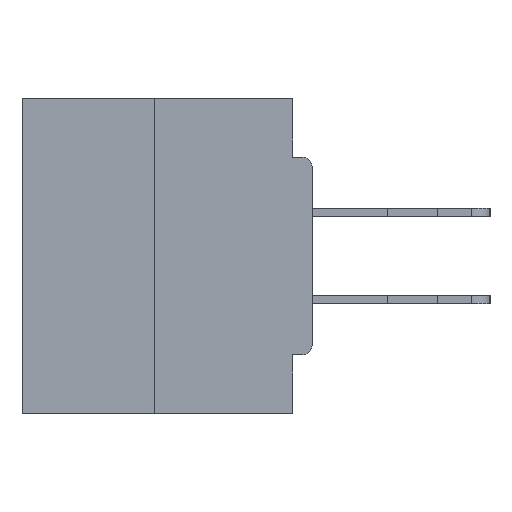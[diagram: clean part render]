
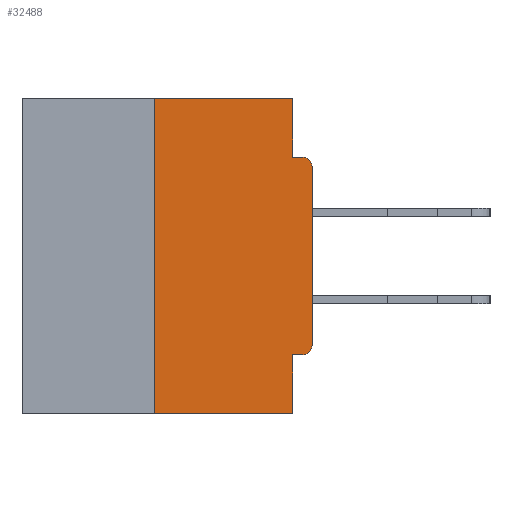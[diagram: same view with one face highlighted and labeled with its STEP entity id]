
A CAD part, left-side view. The second image highlights one B-rep face of the part: STEP entity #32488.
In plain terms, the highlighted planar face has unit normal (-1, 0, 0).
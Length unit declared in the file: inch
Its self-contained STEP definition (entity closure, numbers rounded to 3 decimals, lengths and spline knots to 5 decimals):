
#853 = FACE_OUTER_BOUND ( 'NONE', #29812, .T. ) ;
#1181 = VECTOR ( 'NONE', #7171, 39.37008 ) ;
#1456 = DIRECTION ( 'NONE',  ( 1., 0., 0. ) ) ;
#1654 = LINE ( 'NONE', #13604, #20247 ) ;
#1739 = CARTESIAN_POINT ( 'NONE',  ( 0., 0., 0. ) ) ;
#1899 = VECTOR ( 'NONE', #14951, 39.37008 ) ;
#1932 = VECTOR ( 'NONE', #18897, 39.37008 ) ;
#2019 = ORIENTED_EDGE ( 'NONE', *, *, #27860, .T. ) ;
#2384 = CARTESIAN_POINT ( 'NONE',  ( 0., 0.031, 0. ) ) ;
#3066 = CARTESIAN_POINT ( 'NONE',  ( 0., 0., -0.0935 ) ) ;
#3113 = CARTESIAN_POINT ( 'NONE',  ( 0., 0.015, -0.0935 ) ) ;
#3403 = ORIENTED_EDGE ( 'NONE', *, *, #8009, .T. ) ;
#4052 = ORIENTED_EDGE ( 'NONE', *, *, #5361, .F. ) ;
#4895 = VERTEX_POINT ( 'NONE', #2384 ) ;
#4952 = VECTOR ( 'NONE', #25074, 39.37008 ) ;
#5238 = VECTOR ( 'NONE', #13151, 39.37008 ) ;
#5361 = EDGE_CURVE ( 'NONE', #12038, #23537, #13809, .T. ) ;
#5390 = ORIENTED_EDGE ( 'NONE', *, *, #16022, .T. ) ;
#5860 = AXIS2_PLACEMENT_3D ( 'NONE', #29175, #13803, #16072 ) ;
#5918 = CARTESIAN_POINT ( 'NONE',  ( 0., 0.031, -0.4065 ) ) ;
#7171 = DIRECTION ( 'NONE',  ( 0., 1., 0. ) ) ;
#7186 = VERTEX_POINT ( 'NONE', #13687 ) ;
#7511 = ORIENTED_EDGE ( 'NONE', *, *, #31062, .F. ) ;
#7929 = CIRCLE ( 'NONE', #12005, 0.015 ) ;
#8009 = EDGE_CURVE ( 'NONE', #15146, #13964, #25191, .T. ) ;
#8881 = DIRECTION ( 'NONE',  ( 0., 0., -1. ) ) ;
#9315 = ORIENTED_EDGE ( 'NONE', *, *, #19777, .F. ) ;
#10478 = VERTEX_POINT ( 'NONE', #12437 ) ;
#11293 = LINE ( 'NONE', #22627, #1181 ) ;
#11487 = CARTESIAN_POINT ( 'NONE',  ( 0., 0.015, -0.3915 ) ) ;
#12005 = AXIS2_PLACEMENT_3D ( 'NONE', #11487, #16688, #8881 ) ;
#12038 = VERTEX_POINT ( 'NONE', #17807 ) ;
#12060 = LINE ( 'NONE', #24459, #1932 ) ;
#12196 = VERTEX_POINT ( 'NONE', #31091 ) ;
#12437 = CARTESIAN_POINT ( 'NONE',  ( 0., 0., -0.3915 ) ) ;
#13151 = DIRECTION ( 'NONE',  ( 0., -1., 0. ) ) ;
#13604 = CARTESIAN_POINT ( 'NONE',  ( 0., 0.031, -0.5 ) ) ;
#13687 = CARTESIAN_POINT ( 'NONE',  ( 0., 0.25, 0. ) ) ;
#13803 = DIRECTION ( 'NONE',  ( -1., 0., 0. ) ) ;
#13809 = LINE ( 'NONE', #3066, #16246 ) ;
#13826 = CARTESIAN_POINT ( 'NONE',  ( 0., 0.25, 0. ) ) ;
#13964 = VERTEX_POINT ( 'NONE', #17388 ) ;
#14284 = EDGE_CURVE ( 'NONE', #4895, #12038, #12060, .T. ) ;
#14951 = DIRECTION ( 'NONE',  ( 0., 0., 1. ) ) ;
#15146 = VERTEX_POINT ( 'NONE', #29995 ) ;
#15841 = DIRECTION ( 'NONE',  ( 0., -1., 0. ) ) ;
#16022 = EDGE_CURVE ( 'NONE', #12196, #23537, #31700, .T. ) ;
#16072 = DIRECTION ( 'NONE',  ( 0., 0., -1. ) ) ;
#16246 = VECTOR ( 'NONE', #15841, 39.37008 ) ;
#16395 = LINE ( 'NONE', #13826, #25697 ) ;
#16688 = DIRECTION ( 'NONE',  ( -1., 0., 0. ) ) ;
#17388 = CARTESIAN_POINT ( 'NONE',  ( 0., 0.031, -0.5 ) ) ;
#17807 = CARTESIAN_POINT ( 'NONE',  ( 0., 0.031, -0.0935 ) ) ;
#18897 = DIRECTION ( 'NONE',  ( 0., 0., -1. ) ) ;
#19366 = EDGE_CURVE ( 'NONE', #26482, #10478, #7929, .T. ) ;
#19777 = EDGE_CURVE ( 'NONE', #15146, #7186, #16395, .T. ) ;
#20247 = VECTOR ( 'NONE', #31413, 39.37008 ) ;
#20507 = VERTEX_POINT ( 'NONE', #5918 ) ;
#21269 = LINE ( 'NONE', #1739, #1899 ) ;
#21563 = PLANE ( 'NONE',  #22716 ) ;
#22377 = ORIENTED_EDGE ( 'NONE', *, *, #19366, .T. ) ;
#22627 = CARTESIAN_POINT ( 'NONE',  ( 0., 0., -0.4065 ) ) ;
#22716 = AXIS2_PLACEMENT_3D ( 'NONE', #32154, #1456, #24288 ) ;
#22991 = ORIENTED_EDGE ( 'NONE', *, *, #24390, .F. ) ;
#23537 = VERTEX_POINT ( 'NONE', #3113 ) ;
#23901 = DIRECTION ( 'NONE',  ( 0., 0., 1. ) ) ;
#24288 = DIRECTION ( 'NONE',  ( 0., 0., -1. ) ) ;
#24390 = EDGE_CURVE ( 'NONE', #7186, #4895, #28659, .T. ) ;
#24459 = CARTESIAN_POINT ( 'NONE',  ( 0., 0.031, 0. ) ) ;
#25074 = DIRECTION ( 'NONE',  ( 0., -1., 0. ) ) ;
#25191 = LINE ( 'NONE', #32707, #4952 ) ;
#25697 = VECTOR ( 'NONE', #23901, 39.37008 ) ;
#25841 = EDGE_CURVE ( 'NONE', #26482, #20507, #11293, .T. ) ;
#26090 = ORIENTED_EDGE ( 'NONE', *, *, #25841, .F. ) ;
#26482 = VERTEX_POINT ( 'NONE', #27589 ) ;
#27589 = CARTESIAN_POINT ( 'NONE',  ( 0., 0.015, -0.4065 ) ) ;
#27860 = EDGE_CURVE ( 'NONE', #10478, #12196, #21269, .T. ) ;
#28629 = CARTESIAN_POINT ( 'NONE',  ( 0., 0.46, 0. ) ) ;
#28659 = LINE ( 'NONE', #28629, #5238 ) ;
#29175 = CARTESIAN_POINT ( 'NONE',  ( 0., 0.015, -0.1085 ) ) ;
#29812 = EDGE_LOOP ( 'NONE', ( #22991, #9315, #3403, #7511, #26090, #22377, #2019, #5390, #4052, #29945 ) ) ;
#29945 = ORIENTED_EDGE ( 'NONE', *, *, #14284, .F. ) ;
#29995 = CARTESIAN_POINT ( 'NONE',  ( 0., 0.25, -0.5 ) ) ;
#31062 = EDGE_CURVE ( 'NONE', #20507, #13964, #1654, .T. ) ;
#31091 = CARTESIAN_POINT ( 'NONE',  ( 0., 0., -0.1085 ) ) ;
#31413 = DIRECTION ( 'NONE',  ( 0., 0., -1. ) ) ;
#31700 = CIRCLE ( 'NONE', #5860, 0.015 ) ;
#32154 = CARTESIAN_POINT ( 'NONE',  ( 0., 0.46, 0. ) ) ;
#32488 = ADVANCED_FACE ( 'NONE', ( #853 ), #21563, .F. ) ;
#32707 = CARTESIAN_POINT ( 'NONE',  ( 0., 0.46, -0.5 ) ) ;
